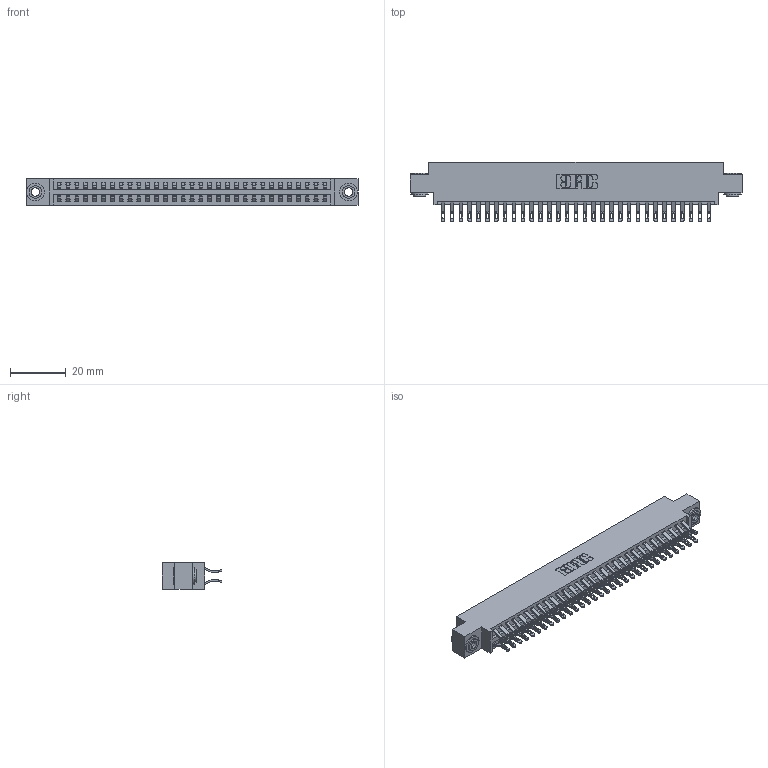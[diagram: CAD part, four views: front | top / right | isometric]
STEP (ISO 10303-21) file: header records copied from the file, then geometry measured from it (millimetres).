
FILE_DESCRIPTION (( 'STEP AP203' ), '1' );
FILE_NAME ('346-062-555-803.STEP', '2022-05-24T14:04:48', ( '' ), ( '' ), 'SwSTEP 2.0', 'SolidWorks 2020', '' );
FILE_SCHEMA (( 'CONFIG_CONTROL_DESIGN' ));
Length unit declared in the file: inch
Products named in the file (4): 345-292-001_555 Tail; 346-062-555-803; 346 Part_0.170 Offset - 0.156 Dia-TH; 345-250-002_345-250-002-102
Assembly tree (65 placements, depth 2):
  346-062-555-803
    346 Part_0.170 Offset - 0.156 Dia-TH
    345-292-001_555 Tail  x62
    345-250-002_345-250-002-102  x2
Bounding box: 119 x 21.46 x 9.4 mm (x, y, z)
Volume: 11545 mm3; surface area: 16765.8 mm2
Topology: 65 solids, 65 shells, 3774 faces, 11799 edges, 7862 vertices
Faces by surface type: plane 2150, cylinder 1616, cone 8
Entity records: 23236 total; most frequent: CARTESIAN_POINT 3863, ORIENTED_EDGE 3758, DIRECTION 3453, EDGE_CURVE 1879, VECTOR 1579, LINE 1579, VERTEX_POINT 1250, AXIS2_PLACEMENT_3D 937
